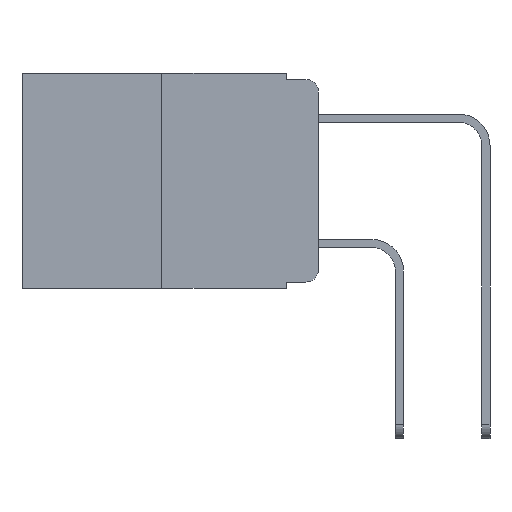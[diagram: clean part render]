
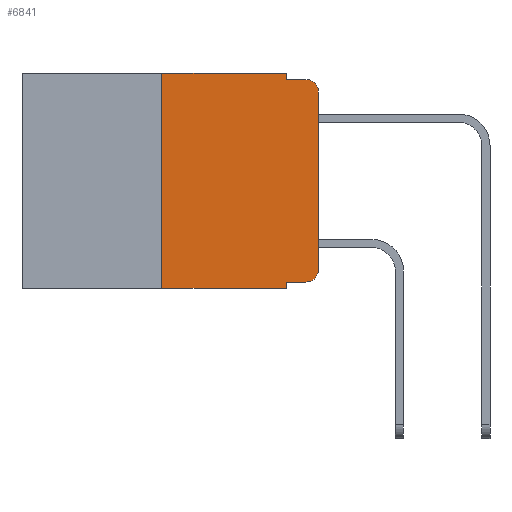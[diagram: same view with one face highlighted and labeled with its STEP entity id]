
A CAD part, left-side view. The second image highlights one B-rep face of the part: STEP entity #6841.
In plain terms, the highlighted planar face has unit normal (-1, 0, 0).
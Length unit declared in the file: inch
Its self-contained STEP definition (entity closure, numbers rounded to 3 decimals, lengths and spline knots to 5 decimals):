
#83 = EDGE_CURVE ( 'NONE', #5793, #12224, #11268, .T. ) ;
#87 = VECTOR ( 'NONE', #2092, 39.37008 ) ;
#161 = ORIENTED_EDGE ( 'NONE', *, *, #6514, .F. ) ;
#220 = LINE ( 'NONE', #899, #10257 ) ;
#249 = CARTESIAN_POINT ( 'NONE',  ( 0., 0.051, -0.343 ) ) ;
#387 = CARTESIAN_POINT ( 'NONE',  ( 0., 0., 0. ) ) ;
#529 = AXIS2_PLACEMENT_3D ( 'NONE', #1553, #8420, #2591 ) ;
#603 = CARTESIAN_POINT ( 'NONE',  ( 0., 0.051, -0.333 ) ) ;
#726 = EDGE_CURVE ( 'NONE', #4895, #11584, #7476, .T. ) ;
#806 = DIRECTION ( 'NONE',  ( 0., 0., -1. ) ) ;
#846 = DIRECTION ( 'NONE',  ( 0., -1., 0. ) ) ;
#858 = CARTESIAN_POINT ( 'NONE',  ( 0., 0.051, -0.01 ) ) ;
#899 = CARTESIAN_POINT ( 'NONE',  ( 0., 0.473, 0. ) ) ;
#905 = LINE ( 'NONE', #4527, #10791 ) ;
#1173 = ORIENTED_EDGE ( 'NONE', *, *, #6273, .F. ) ;
#1178 = VERTEX_POINT ( 'NONE', #1762 ) ;
#1553 = CARTESIAN_POINT ( 'NONE',  ( 0., 0.02, -0.313 ) ) ;
#1762 = CARTESIAN_POINT ( 'NONE',  ( 0., 0.051, 0. ) ) ;
#1825 = VECTOR ( 'NONE', #9795, 39.37008 ) ;
#2092 = DIRECTION ( 'NONE',  ( 0., -1., 0. ) ) ;
#2155 = LINE ( 'NONE', #6162, #1825 ) ;
#2241 = VECTOR ( 'NONE', #11771, 39.37008 ) ;
#2281 = EDGE_CURVE ( 'NONE', #5734, #4333, #905, .T. ) ;
#2292 = CIRCLE ( 'NONE', #529, 0.02 ) ;
#2300 = ORIENTED_EDGE ( 'NONE', *, *, #4195, .F. ) ;
#2311 = ORIENTED_EDGE ( 'NONE', *, *, #726, .F. ) ;
#2591 = DIRECTION ( 'NONE',  ( 0., 0., -1. ) ) ;
#2791 = ORIENTED_EDGE ( 'NONE', *, *, #2281, .T. ) ;
#2833 = EDGE_CURVE ( 'NONE', #11584, #1178, #220, .T. ) ;
#2853 = LINE ( 'NONE', #8902, #87 ) ;
#2892 = CARTESIAN_POINT ( 'NONE',  ( 0., 0.25, 0. ) ) ;
#3058 = VECTOR ( 'NONE', #5429, 39.37008 ) ;
#3360 = CARTESIAN_POINT ( 'NONE',  ( 0., 0.02, -0.03 ) ) ;
#3391 = VERTEX_POINT ( 'NONE', #7465 ) ;
#3813 = PLANE ( 'NONE',  #9533 ) ;
#4195 = EDGE_CURVE ( 'NONE', #3391, #12224, #5576, .T. ) ;
#4333 = VERTEX_POINT ( 'NONE', #4948 ) ;
#4337 = VECTOR ( 'NONE', #5250, 39.37008 ) ;
#4475 = DIRECTION ( 'NONE',  ( 0., -1., 0. ) ) ;
#4527 = CARTESIAN_POINT ( 'NONE',  ( 0., 0.051, -0.333 ) ) ;
#4852 = CARTESIAN_POINT ( 'NONE',  ( 0., 0.25, 0. ) ) ;
#4895 = VERTEX_POINT ( 'NONE', #5675 ) ;
#4948 = CARTESIAN_POINT ( 'NONE',  ( 0., 0.02, -0.333 ) ) ;
#5250 = DIRECTION ( 'NONE',  ( 0., 0., -1. ) ) ;
#5256 = ORIENTED_EDGE ( 'NONE', *, *, #11724, .T. ) ;
#5317 = DIRECTION ( 'NONE',  ( 0., 0., -1. ) ) ;
#5429 = DIRECTION ( 'NONE',  ( 0., 0., 1. ) ) ;
#5571 = CARTESIAN_POINT ( 'NONE',  ( 0., 0., -0.03 ) ) ;
#5576 = LINE ( 'NONE', #858, #8422 ) ;
#5616 = VERTEX_POINT ( 'NONE', #249 ) ;
#5675 = CARTESIAN_POINT ( 'NONE',  ( 0., 0.25, -0.343 ) ) ;
#5680 = LINE ( 'NONE', #387, #3058 ) ;
#5734 = VERTEX_POINT ( 'NONE', #603 ) ;
#5793 = VERTEX_POINT ( 'NONE', #5571 ) ;
#6162 = CARTESIAN_POINT ( 'NONE',  ( 0., 0.051, 0. ) ) ;
#6273 = EDGE_CURVE ( 'NONE', #5734, #5616, #2155, .T. ) ;
#6323 = ORIENTED_EDGE ( 'NONE', *, *, #7837, .T. ) ;
#6514 = EDGE_CURVE ( 'NONE', #1178, #3391, #9397, .T. ) ;
#6805 = DIRECTION ( 'NONE',  ( 1., 0., 0. ) ) ;
#6841 = ADVANCED_FACE ( 'NONE', ( #9944 ), #3813, .F. ) ;
#6970 = ORIENTED_EDGE ( 'NONE', *, *, #2833, .F. ) ;
#7327 = EDGE_CURVE ( 'NONE', #4333, #12178, #2292, .T. ) ;
#7465 = CARTESIAN_POINT ( 'NONE',  ( 0., 0.051, -0.01 ) ) ;
#7476 = LINE ( 'NONE', #4852, #2241 ) ;
#7837 = EDGE_CURVE ( 'NONE', #12178, #5793, #5680, .T. ) ;
#8201 = EDGE_LOOP ( 'NONE', ( #6323, #9382, #2300, #161, #6970, #2311, #5256, #1173, #2791, #8271 ) ) ;
#8233 = CARTESIAN_POINT ( 'NONE',  ( 0., 0., -0.313 ) ) ;
#8271 = ORIENTED_EDGE ( 'NONE', *, *, #7327, .T. ) ;
#8420 = DIRECTION ( 'NONE',  ( -1., 0., 0. ) ) ;
#8422 = VECTOR ( 'NONE', #846, 39.37008 ) ;
#8715 = DIRECTION ( 'NONE',  ( -1., 0., 0. ) ) ;
#8902 = CARTESIAN_POINT ( 'NONE',  ( 0., 0.473, -0.343 ) ) ;
#9382 = ORIENTED_EDGE ( 'NONE', *, *, #83, .T. ) ;
#9397 = LINE ( 'NONE', #9928, #4337 ) ;
#9533 = AXIS2_PLACEMENT_3D ( 'NONE', #12139, #6805, #806 ) ;
#9795 = DIRECTION ( 'NONE',  ( 0., 0., -1. ) ) ;
#9928 = CARTESIAN_POINT ( 'NONE',  ( 0., 0.051, 0. ) ) ;
#9944 = FACE_OUTER_BOUND ( 'NONE', #8201, .T. ) ;
#10219 = CARTESIAN_POINT ( 'NONE',  ( 0., 0.02, -0.01 ) ) ;
#10257 = VECTOR ( 'NONE', #12022, 39.37008 ) ;
#10791 = VECTOR ( 'NONE', #4475, 39.37008 ) ;
#11268 = CIRCLE ( 'NONE', #11532, 0.02 ) ;
#11532 = AXIS2_PLACEMENT_3D ( 'NONE', #3360, #8715, #5317 ) ;
#11584 = VERTEX_POINT ( 'NONE', #2892 ) ;
#11724 = EDGE_CURVE ( 'NONE', #4895, #5616, #2853, .T. ) ;
#11771 = DIRECTION ( 'NONE',  ( 0., 0., 1. ) ) ;
#12022 = DIRECTION ( 'NONE',  ( 0., -1., 0. ) ) ;
#12139 = CARTESIAN_POINT ( 'NONE',  ( 0., 0.473, 0. ) ) ;
#12178 = VERTEX_POINT ( 'NONE', #8233 ) ;
#12224 = VERTEX_POINT ( 'NONE', #10219 ) ;
